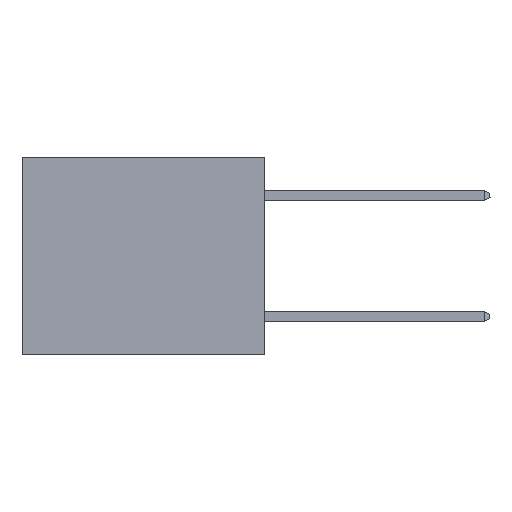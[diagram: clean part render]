
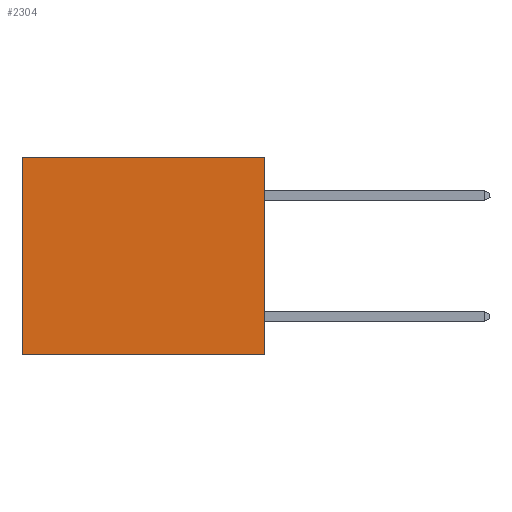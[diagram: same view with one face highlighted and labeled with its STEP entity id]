
A CAD part, left-side view. The second image highlights one B-rep face of the part: STEP entity #2304.
In plain terms, the highlighted planar face has unit normal (-1, 0, 0).
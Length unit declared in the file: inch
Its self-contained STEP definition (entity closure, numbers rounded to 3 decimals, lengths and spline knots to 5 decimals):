
#354 = LINE ( 'NONE', #21984, #8067 ) ;
#865 = LINE ( 'NONE', #14949, #24448 ) ;
#1538 = EDGE_CURVE ( 'NONE', #26401, #5531, #354, .T. ) ;
#2304 = ADVANCED_FACE ( 'NONE', ( #9753 ), #11236, .F. ) ;
#2502 = CARTESIAN_POINT ( 'NONE',  ( 0.3165, 0.6, 0. ) ) ;
#2962 = VECTOR ( 'NONE', #22556, 39.37008 ) ;
#2987 = VERTEX_POINT ( 'NONE', #2502 ) ;
#3894 = ORIENTED_EDGE ( 'NONE', *, *, #3962, .F. ) ;
#3962 = EDGE_CURVE ( 'NONE', #5531, #5292, #13016, .T. ) ;
#4963 = DIRECTION ( 'NONE',  ( 0., 0., -1. ) ) ;
#5026 = EDGE_LOOP ( 'NONE', ( #19050, #3894, #8136, #26680 ) ) ;
#5292 = VERTEX_POINT ( 'NONE', #17465 ) ;
#5531 = VERTEX_POINT ( 'NONE', #24885 ) ;
#8067 = VECTOR ( 'NONE', #10879, 39.37008 ) ;
#8136 = ORIENTED_EDGE ( 'NONE', *, *, #1538, .F. ) ;
#9753 = FACE_OUTER_BOUND ( 'NONE', #5026, .T. ) ;
#10879 = DIRECTION ( 'NONE',  ( 0., 0., -1. ) ) ;
#11195 = AXIS2_PLACEMENT_3D ( 'NONE', #20220, #24272, #4963 ) ;
#11236 = PLANE ( 'NONE',  #11195 ) ;
#12056 = CARTESIAN_POINT ( 'NONE',  ( 0.3165, 0., 0. ) ) ;
#13016 = LINE ( 'NONE', #18205, #2962 ) ;
#14747 = LINE ( 'NONE', #20844, #24844 ) ;
#14949 = CARTESIAN_POINT ( 'NONE',  ( 0.3165, 0., 0. ) ) ;
#16335 = DIRECTION ( 'NONE',  ( 0., 0., -1. ) ) ;
#16944 = DIRECTION ( 'NONE',  ( 0., 1., 0. ) ) ;
#17465 = CARTESIAN_POINT ( 'NONE',  ( 0.3165, 0.6, -0.49 ) ) ;
#18205 = CARTESIAN_POINT ( 'NONE',  ( 0.3165, 0., -0.49 ) ) ;
#19050 = ORIENTED_EDGE ( 'NONE', *, *, #20746, .T. ) ;
#20220 = CARTESIAN_POINT ( 'NONE',  ( 0.3165, 0., -0.49 ) ) ;
#20746 = EDGE_CURVE ( 'NONE', #2987, #5292, #14747, .T. ) ;
#20844 = CARTESIAN_POINT ( 'NONE',  ( 0.3165, 0.6, -0.49 ) ) ;
#21984 = CARTESIAN_POINT ( 'NONE',  ( 0.3165, 0., -0.49 ) ) ;
#22402 = EDGE_CURVE ( 'NONE', #26401, #2987, #865, .T. ) ;
#22556 = DIRECTION ( 'NONE',  ( 0., 1., 0. ) ) ;
#24272 = DIRECTION ( 'NONE',  ( 1., 0., 0. ) ) ;
#24448 = VECTOR ( 'NONE', #16944, 39.37008 ) ;
#24844 = VECTOR ( 'NONE', #16335, 39.37008 ) ;
#24885 = CARTESIAN_POINT ( 'NONE',  ( 0.3165, 0., -0.49 ) ) ;
#26401 = VERTEX_POINT ( 'NONE', #12056 ) ;
#26680 = ORIENTED_EDGE ( 'NONE', *, *, #22402, .T. ) ;
